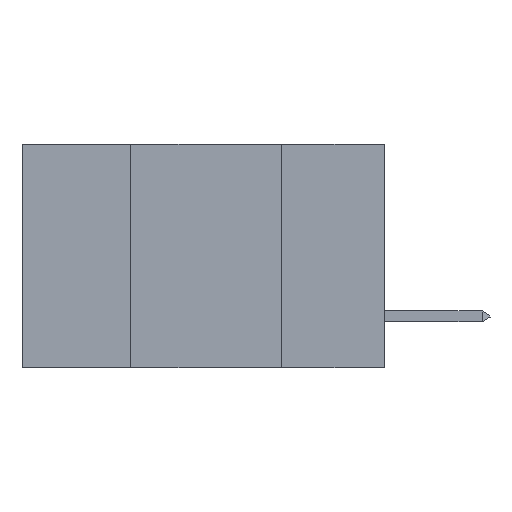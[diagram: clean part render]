
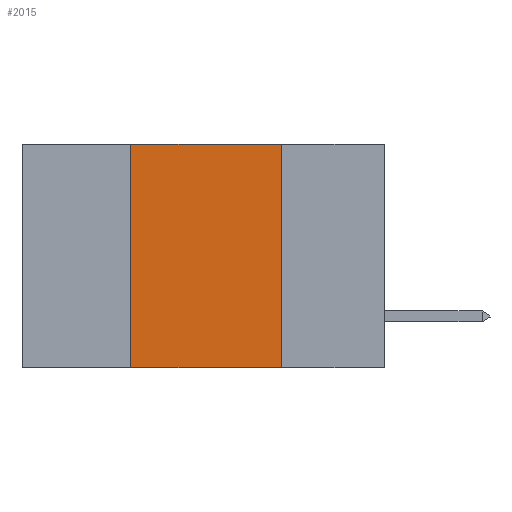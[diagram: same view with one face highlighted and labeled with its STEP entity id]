
A CAD part, left-side view. The second image highlights one B-rep face of the part: STEP entity #2015.
In plain terms, the highlighted planar face has unit normal (-1, 0, 0).
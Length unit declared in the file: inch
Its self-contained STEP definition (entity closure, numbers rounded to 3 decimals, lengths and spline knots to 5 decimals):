
#1271 = EDGE_LOOP ( 'NONE', ( #32134, #9596, #21209, #15244 ) ) ;
#1988 = VERTEX_POINT ( 'NONE', #33616 ) ;
#2015 = ADVANCED_FACE ( 'NONE', ( #29282 ), #16318, .F. ) ;
#2438 = VECTOR ( 'NONE', #19283, 39.37008 ) ;
#3218 = VERTEX_POINT ( 'NONE', #13031 ) ;
#3261 = LINE ( 'NONE', #7624, #2438 ) ;
#3410 = DIRECTION ( 'NONE',  ( 0., -1., 0. ) ) ;
#7165 = VERTEX_POINT ( 'NONE', #12883 ) ;
#7380 = VERTEX_POINT ( 'NONE', #36150 ) ;
#7624 = CARTESIAN_POINT ( 'NONE',  ( 0., 0.17, 0. ) ) ;
#9505 = CARTESIAN_POINT ( 'NONE',  ( 0., 0.42, 0. ) ) ;
#9596 = ORIENTED_EDGE ( 'NONE', *, *, #23132, .F. ) ;
#11791 = EDGE_CURVE ( 'NONE', #1988, #3218, #26368, .T. ) ;
#12883 = CARTESIAN_POINT ( 'NONE',  ( 0., 0.17, 0. ) ) ;
#13031 = CARTESIAN_POINT ( 'NONE',  ( 0., 0.42, 0. ) ) ;
#13550 = EDGE_CURVE ( 'NONE', #7165, #7380, #3261, .T. ) ;
#15244 = ORIENTED_EDGE ( 'NONE', *, *, #27866, .T. ) ;
#15251 = LINE ( 'NONE', #33312, #16746 ) ;
#15729 = LINE ( 'NONE', #29513, #32896 ) ;
#16318 = PLANE ( 'NONE',  #17746 ) ;
#16746 = VECTOR ( 'NONE', #34765, 39.37008 ) ;
#17746 = AXIS2_PLACEMENT_3D ( 'NONE', #22375, #25027, #28046 ) ;
#18368 = DIRECTION ( 'NONE',  ( 0., 0., 1. ) ) ;
#19283 = DIRECTION ( 'NONE',  ( 0., 0., -1. ) ) ;
#19294 = VECTOR ( 'NONE', #18368, 39.37008 ) ;
#21209 = ORIENTED_EDGE ( 'NONE', *, *, #11791, .F. ) ;
#22375 = CARTESIAN_POINT ( 'NONE',  ( 0., 0.6, 0. ) ) ;
#23132 = EDGE_CURVE ( 'NONE', #3218, #7165, #15729, .T. ) ;
#25027 = DIRECTION ( 'NONE',  ( 1., 0., 0. ) ) ;
#26368 = LINE ( 'NONE', #9505, #19294 ) ;
#27866 = EDGE_CURVE ( 'NONE', #1988, #7380, #15251, .T. ) ;
#28046 = DIRECTION ( 'NONE',  ( 0., 0., -1. ) ) ;
#29282 = FACE_OUTER_BOUND ( 'NONE', #1271, .T. ) ;
#29513 = CARTESIAN_POINT ( 'NONE',  ( 0., 0.6, 0. ) ) ;
#32134 = ORIENTED_EDGE ( 'NONE', *, *, #13550, .F. ) ;
#32896 = VECTOR ( 'NONE', #3410, 39.37008 ) ;
#33312 = CARTESIAN_POINT ( 'NONE',  ( 0., 0.6, -0.37 ) ) ;
#33616 = CARTESIAN_POINT ( 'NONE',  ( 0., 0.42, -0.37 ) ) ;
#34765 = DIRECTION ( 'NONE',  ( 0., -1., 0. ) ) ;
#36150 = CARTESIAN_POINT ( 'NONE',  ( 0., 0.17, -0.37 ) ) ;
